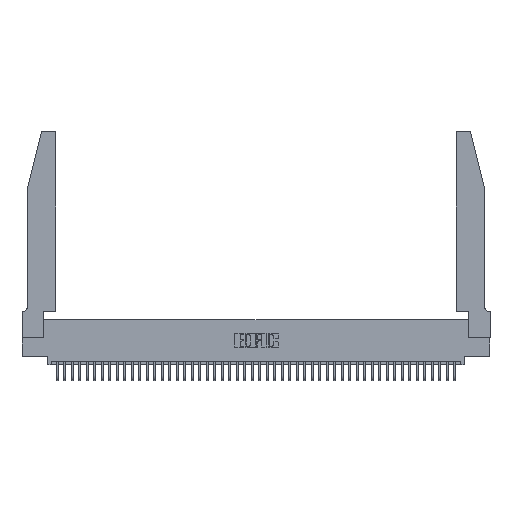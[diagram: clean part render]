
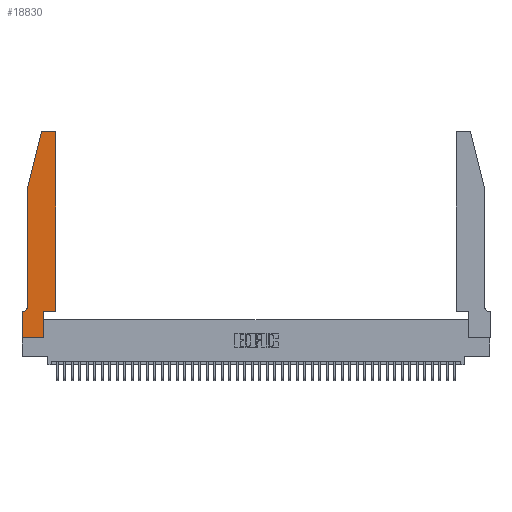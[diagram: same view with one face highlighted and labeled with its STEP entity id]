
A CAD part, top view. The second image highlights one B-rep face of the part: STEP entity #18830.
In plain terms, the highlighted planar face has unit normal (0, 0, 1).
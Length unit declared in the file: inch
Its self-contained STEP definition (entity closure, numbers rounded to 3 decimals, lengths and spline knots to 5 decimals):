
#482 = CARTESIAN_POINT ( 'NONE',  ( 0.0755, 2., 0.37 ) ) ;
#662 = CARTESIAN_POINT ( 'NONE',  ( 0.4505, 0.35, 0.37 ) ) ;
#2326 = EDGE_CURVE ( 'NONE', #38636, #22799, #46620, .T. ) ;
#2362 = CARTESIAN_POINT ( 'NONE',  ( 0.0755, 2., 0.37 ) ) ;
#2475 = ORIENTED_EDGE ( 'NONE', *, *, #13920, .T. ) ;
#3161 = CARTESIAN_POINT ( 'NONE',  ( 0.0755, 0.42, 0.37 ) ) ;
#3443 = EDGE_CURVE ( 'NONE', #3527, #38636, #43541, .T. ) ;
#3527 = VERTEX_POINT ( 'NONE', #34428 ) ;
#4022 = CARTESIAN_POINT ( 'NONE',  ( 0.2865, 0.35, 0.37 ) ) ;
#4048 = VERTEX_POINT ( 'NONE', #16744 ) ;
#4207 = VERTEX_POINT ( 'NONE', #33738 ) ;
#4393 = DIRECTION ( 'NONE',  ( 0., 0., 1. ) ) ;
#4880 = VERTEX_POINT ( 'NONE', #26884 ) ;
#5708 = CIRCLE ( 'NONE', #9444, 0.03 ) ;
#6203 = EDGE_CURVE ( 'NONE', #45311, #3527, #11269, .T. ) ;
#6638 = CARTESIAN_POINT ( 'NONE',  ( 0., 0., 0.37 ) ) ;
#6948 = VECTOR ( 'NONE', #24579, 39.37008 ) ;
#7122 = ORIENTED_EDGE ( 'NONE', *, *, #40213, .T. ) ;
#8268 = CARTESIAN_POINT ( 'NONE',  ( 0., 0.35, 0.37 ) ) ;
#8496 = DIRECTION ( 'NONE',  ( 1., 0., 0. ) ) ;
#8873 = ORIENTED_EDGE ( 'NONE', *, *, #14209, .T. ) ;
#9043 = VECTOR ( 'NONE', #38234, 39.37008 ) ;
#9299 = CARTESIAN_POINT ( 'NONE',  ( 0.2605, 2.75, 0.37 ) ) ;
#9444 = AXIS2_PLACEMENT_3D ( 'NONE', #26043, #25400, #21714 ) ;
#10754 = LINE ( 'NONE', #23863, #9043 ) ;
#11269 = LINE ( 'NONE', #482, #43291 ) ;
#11297 = VECTOR ( 'NONE', #15344, 39.37008 ) ;
#11717 = DIRECTION ( 'NONE',  ( 1., 0., 0. ) ) ;
#11850 = ORIENTED_EDGE ( 'NONE', *, *, #13066, .T. ) ;
#12261 = DIRECTION ( 'NONE',  ( 1., 0., 0. ) ) ;
#12414 = LINE ( 'NONE', #6638, #38183 ) ;
#13066 = EDGE_CURVE ( 'NONE', #30438, #18174, #5708, .T. ) ;
#13920 = EDGE_CURVE ( 'NONE', #4207, #22194, #12414, .T. ) ;
#13977 = DIRECTION ( 'NONE',  ( 1., 0., 0. ) ) ;
#14209 = EDGE_CURVE ( 'NONE', #18174, #19120, #38793, .T. ) ;
#15068 = VECTOR ( 'NONE', #36784, 39.37008 ) ;
#15344 = DIRECTION ( 'NONE',  ( -1., 0., 0. ) ) ;
#16478 = CARTESIAN_POINT ( 'NONE',  ( 0.4505, 2.72, 0.37 ) ) ;
#16744 = CARTESIAN_POINT ( 'NONE',  ( 0.2865, 0.35, 0.37 ) ) ;
#17151 = EDGE_LOOP ( 'NONE', ( #8873, #26576, #32552, #36857, #27847, #7122, #17564, #2475, #22690, #33754, #29229, #11850 ) ) ;
#17564 = ORIENTED_EDGE ( 'NONE', *, *, #40835, .T. ) ;
#17903 = CARTESIAN_POINT ( 'NONE',  ( 0.0755, 0.35, 0.37 ) ) ;
#18174 = VERTEX_POINT ( 'NONE', #29240 ) ;
#18755 = LINE ( 'NONE', #17903, #11297 ) ;
#18830 = ADVANCED_FACE ( 'NONE', ( #24876 ), #21098, .T. ) ;
#19120 = VERTEX_POINT ( 'NONE', #19483 ) ;
#19483 = CARTESIAN_POINT ( 'NONE',  ( 0.284, 2.75, 0.37 ) ) ;
#21098 = PLANE ( 'NONE',  #42794 ) ;
#21714 = DIRECTION ( 'NONE',  ( 1., 0., 0. ) ) ;
#22194 = VERTEX_POINT ( 'NONE', #26819 ) ;
#22690 = ORIENTED_EDGE ( 'NONE', *, *, #30155, .T. ) ;
#22799 = VERTEX_POINT ( 'NONE', #30736 ) ;
#22953 = CIRCLE ( 'NONE', #41075, 0.03 ) ;
#23863 = CARTESIAN_POINT ( 'NONE',  ( 0.4505, 0.35, 0.37 ) ) ;
#24373 = CARTESIAN_POINT ( 'NONE',  ( 0., 0., 0.37 ) ) ;
#24500 = DIRECTION ( 'NONE',  ( -1., 0., 0. ) ) ;
#24579 = DIRECTION ( 'NONE',  ( 0., -1., 0. ) ) ;
#24876 = FACE_OUTER_BOUND ( 'NONE', #17151, .T. ) ;
#25400 = DIRECTION ( 'NONE',  ( 0., 0., 1. ) ) ;
#25973 = CARTESIAN_POINT ( 'NONE',  ( 0.284, 2.72, 0.37 ) ) ;
#26043 = CARTESIAN_POINT ( 'NONE',  ( 0.4205, 2.72, 0.37 ) ) ;
#26576 = ORIENTED_EDGE ( 'NONE', *, *, #37576, .T. ) ;
#26819 = CARTESIAN_POINT ( 'NONE',  ( 0.2865, 0., 0.37 ) ) ;
#26884 = CARTESIAN_POINT ( 'NONE',  ( 0.4505, 0.35, 0.37 ) ) ;
#27331 = EDGE_CURVE ( 'NONE', #4048, #4880, #35474, .T. ) ;
#27847 = ORIENTED_EDGE ( 'NONE', *, *, #2326, .T. ) ;
#28757 = CARTESIAN_POINT ( 'NONE',  ( 0.0055, 0.42, 0.37 ) ) ;
#29229 = ORIENTED_EDGE ( 'NONE', *, *, #33239, .T. ) ;
#29240 = CARTESIAN_POINT ( 'NONE',  ( 0.4205, 2.75, 0.37 ) ) ;
#29532 = LINE ( 'NONE', #24373, #35267 ) ;
#29997 = CARTESIAN_POINT ( 'NONE',  ( 0.25487, 2.72718, 0.37 ) ) ;
#30155 = EDGE_CURVE ( 'NONE', #22194, #4048, #45954, .T. ) ;
#30438 = VERTEX_POINT ( 'NONE', #16478 ) ;
#30736 = CARTESIAN_POINT ( 'NONE',  ( 0.0055, 0.35, 0.37 ) ) ;
#30895 = VECTOR ( 'NONE', #8496, 39.37008 ) ;
#31692 = DIRECTION ( 'NONE',  ( 0., -1., 0. ) ) ;
#32552 = ORIENTED_EDGE ( 'NONE', *, *, #6203, .T. ) ;
#33191 = DIRECTION ( 'NONE',  ( 0., 0., -1. ) ) ;
#33239 = EDGE_CURVE ( 'NONE', #4880, #30438, #10754, .T. ) ;
#33738 = CARTESIAN_POINT ( 'NONE',  ( 0., 0., 0.37 ) ) ;
#33754 = ORIENTED_EDGE ( 'NONE', *, *, #27331, .T. ) ;
#34163 = VECTOR ( 'NONE', #24500, 39.37008 ) ;
#34428 = CARTESIAN_POINT ( 'NONE',  ( 0.0755, 2., 0.37 ) ) ;
#34697 = VERTEX_POINT ( 'NONE', #8268 ) ;
#35267 = VECTOR ( 'NONE', #31692, 39.37008 ) ;
#35474 = LINE ( 'NONE', #662, #30895 ) ;
#36784 = DIRECTION ( 'NONE',  ( 0., 1., 0. ) ) ;
#36857 = ORIENTED_EDGE ( 'NONE', *, *, #3443, .T. ) ;
#37576 = EDGE_CURVE ( 'NONE', #19120, #45311, #22953, .T. ) ;
#38183 = VECTOR ( 'NONE', #13977, 39.37008 ) ;
#38234 = DIRECTION ( 'NONE',  ( 0., 1., 0. ) ) ;
#38596 = AXIS2_PLACEMENT_3D ( 'NONE', #28757, #33191, #46251 ) ;
#38636 = VERTEX_POINT ( 'NONE', #3161 ) ;
#38793 = LINE ( 'NONE', #9299, #34163 ) ;
#40213 = EDGE_CURVE ( 'NONE', #22799, #34697, #18755, .T. ) ;
#40277 = DIRECTION ( 'NONE',  ( -0.239, -0.971, 0. ) ) ;
#40835 = EDGE_CURVE ( 'NONE', #34697, #4207, #29532, .T. ) ;
#40927 = DIRECTION ( 'NONE',  ( 0., 0., 1. ) ) ;
#41075 = AXIS2_PLACEMENT_3D ( 'NONE', #25973, #4393, #11717 ) ;
#42794 = AXIS2_PLACEMENT_3D ( 'NONE', #43853, #40927, #12261 ) ;
#43291 = VECTOR ( 'NONE', #40277, 39.37008 ) ;
#43541 = LINE ( 'NONE', #2362, #6948 ) ;
#43853 = CARTESIAN_POINT ( 'NONE',  ( 0., 0.35, 0.37 ) ) ;
#45311 = VERTEX_POINT ( 'NONE', #29997 ) ;
#45954 = LINE ( 'NONE', #4022, #15068 ) ;
#46251 = DIRECTION ( 'NONE',  ( -1., 0., 0. ) ) ;
#46620 = CIRCLE ( 'NONE', #38596, 0.07 ) ;
